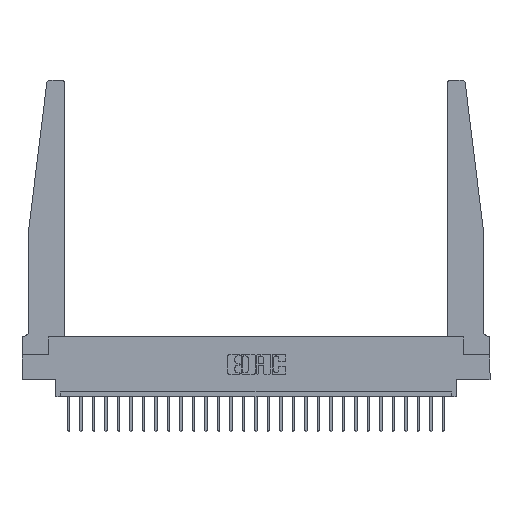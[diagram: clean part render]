
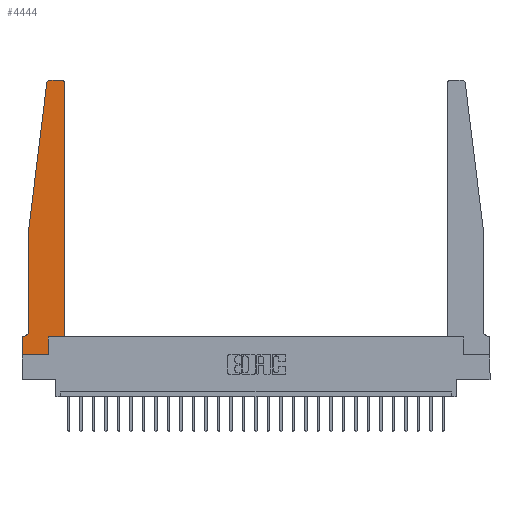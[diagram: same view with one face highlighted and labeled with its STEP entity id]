
A CAD part, top view. The second image highlights one B-rep face of the part: STEP entity #4444.
In plain terms, the highlighted planar face has unit normal (0, 0, 1).
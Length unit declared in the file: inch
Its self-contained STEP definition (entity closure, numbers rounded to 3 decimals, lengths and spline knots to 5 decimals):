
#508 = ORIENTED_EDGE ( 'NONE', *, *, #7807, .T. ) ;
#625 = EDGE_LOOP ( 'NONE', ( #10782, #24775, #23737, #12383, #6452, #21474, #19801, #24273, #508, #15521, #7440, #11717 ) ) ;
#1525 = CARTESIAN_POINT ( 'NONE',  ( 0.395, 2.72, 0.37 ) ) ;
#1667 = AXIS2_PLACEMENT_3D ( 'NONE', #6506, #8773, #2760 ) ;
#2022 = EDGE_CURVE ( 'NONE', #9186, #20017, #14570, .T. ) ;
#2147 = CARTESIAN_POINT ( 'NONE',  ( 0.27653, 2.75, 0.37 ) ) ;
#2467 = VECTOR ( 'NONE', #5396, 39.37008 ) ;
#2760 = DIRECTION ( 'NONE',  ( 1., 0., 0. ) ) ;
#2886 = AXIS2_PLACEMENT_3D ( 'NONE', #18927, #4841, #7091 ) ;
#3070 = CARTESIAN_POINT ( 'NONE',  ( 0.25, 2.75, 0.37 ) ) ;
#4006 = CARTESIAN_POINT ( 'NONE',  ( 0., 0.1875, 0.37 ) ) ;
#4007 = CARTESIAN_POINT ( 'NONE',  ( 0.015, 0.1875, 0.37 ) ) ;
#4085 = CARTESIAN_POINT ( 'NONE',  ( 0.425, 0.18, 0.37 ) ) ;
#4384 = VECTOR ( 'NONE', #7487, 39.37008 ) ;
#4444 = ADVANCED_FACE ( 'NONE', ( #12600 ), #25654, .T. ) ;
#4841 = DIRECTION ( 'NONE',  ( 0., 0., -1. ) ) ;
#5156 = EDGE_CURVE ( 'NONE', #14250, #10541, #24199, .T. ) ;
#5257 = VERTEX_POINT ( 'NONE', #4085 ) ;
#5294 = LINE ( 'NONE', #23390, #18319 ) ;
#5396 = DIRECTION ( 'NONE',  ( 0., -1., 0. ) ) ;
#5636 = EDGE_CURVE ( 'NONE', #18370, #9739, #24785, .T. ) ;
#6045 = EDGE_CURVE ( 'NONE', #23744, #9186, #22267, .T. ) ;
#6452 = ORIENTED_EDGE ( 'NONE', *, *, #2022, .T. ) ;
#6506 = CARTESIAN_POINT ( 'NONE',  ( 0.27653, 2.72, 0.37 ) ) ;
#6831 = DIRECTION ( 'NONE',  ( 0., 1., 0. ) ) ;
#7091 = DIRECTION ( 'NONE',  ( -1., 0., 0. ) ) ;
#7416 = EDGE_CURVE ( 'NONE', #20017, #22170, #16360, .T. ) ;
#7440 = ORIENTED_EDGE ( 'NONE', *, *, #16247, .T. ) ;
#7487 = DIRECTION ( 'NONE',  ( 1., 0., 0. ) ) ;
#7807 = EDGE_CURVE ( 'NONE', #10541, #13994, #12929, .T. ) ;
#7838 = DIRECTION ( 'NONE',  ( 0., 0., 1. ) ) ;
#7997 = VECTOR ( 'NONE', #18767, 39.37008 ) ;
#8141 = EDGE_CURVE ( 'NONE', #9739, #23744, #11986, .T. ) ;
#8773 = DIRECTION ( 'NONE',  ( 0., 0., 1. ) ) ;
#9186 = VERTEX_POINT ( 'NONE', #20401 ) ;
#9189 = VECTOR ( 'NONE', #20879, 39.37008 ) ;
#9529 = DIRECTION ( 'NONE',  ( 1., 0., 0. ) ) ;
#9532 = VECTOR ( 'NONE', #18486, 39.37008 ) ;
#9739 = VERTEX_POINT ( 'NONE', #24891 ) ;
#10285 = EDGE_CURVE ( 'NONE', #23157, #18370, #13423, .T. ) ;
#10321 = VECTOR ( 'NONE', #16860, 39.37008 ) ;
#10541 = VERTEX_POINT ( 'NONE', #16503 ) ;
#10782 = ORIENTED_EDGE ( 'NONE', *, *, #10285, .T. ) ;
#11386 = VERTEX_POINT ( 'NONE', #14234 ) ;
#11481 = CARTESIAN_POINT ( 'NONE',  ( 0., 0., 0.37 ) ) ;
#11717 = ORIENTED_EDGE ( 'NONE', *, *, #21036, .T. ) ;
#11986 = LINE ( 'NONE', #12971, #9189 ) ;
#12216 = CARTESIAN_POINT ( 'NONE',  ( 0., 0., 0.37 ) ) ;
#12383 = ORIENTED_EDGE ( 'NONE', *, *, #6045, .T. ) ;
#12434 = EDGE_CURVE ( 'NONE', #13994, #5257, #19121, .T. ) ;
#12557 = CARTESIAN_POINT ( 'NONE',  ( 0.2605, 0.18, 0.37 ) ) ;
#12559 = CARTESIAN_POINT ( 'NONE',  ( 0., 0.1875, 0.37 ) ) ;
#12600 = FACE_OUTER_BOUND ( 'NONE', #625, .T. ) ;
#12843 = CARTESIAN_POINT ( 'NONE',  ( 0.425, 0.18, 0.37 ) ) ;
#12929 = LINE ( 'NONE', #12557, #9532 ) ;
#12971 = CARTESIAN_POINT ( 'NONE',  ( 0.065, 1.25, 0.37 ) ) ;
#13089 = CARTESIAN_POINT ( 'NONE',  ( 0.2605, 0.18, 0.37 ) ) ;
#13346 = CARTESIAN_POINT ( 'NONE',  ( 0.065, 1.25, 0.37 ) ) ;
#13423 = LINE ( 'NONE', #3070, #10321 ) ;
#13994 = VERTEX_POINT ( 'NONE', #13089 ) ;
#14234 = CARTESIAN_POINT ( 'NONE',  ( 0.425, 2.72, 0.37 ) ) ;
#14250 = VERTEX_POINT ( 'NONE', #12216 ) ;
#14570 = CIRCLE ( 'NONE', #2886, 0.05 ) ;
#14843 = DIRECTION ( 'NONE',  ( -1., 0., 0. ) ) ;
#15164 = CARTESIAN_POINT ( 'NONE',  ( 0.395, 2.75, 0.37 ) ) ;
#15274 = CARTESIAN_POINT ( 'NONE',  ( 0.065, 1.25, 0.37 ) ) ;
#15460 = DIRECTION ( 'NONE',  ( 0., 0., 1. ) ) ;
#15521 = ORIENTED_EDGE ( 'NONE', *, *, #12434, .T. ) ;
#16247 = EDGE_CURVE ( 'NONE', #5257, #11386, #5294, .T. ) ;
#16360 = LINE ( 'NONE', #16748, #17584 ) ;
#16503 = CARTESIAN_POINT ( 'NONE',  ( 0.2605, 0., 0.37 ) ) ;
#16748 = CARTESIAN_POINT ( 'NONE',  ( 0.065, 0.1875, 0.37 ) ) ;
#16860 = DIRECTION ( 'NONE',  ( -1., 0., 0. ) ) ;
#16989 = CIRCLE ( 'NONE', #21179, 0.03 ) ;
#17584 = VECTOR ( 'NONE', #14843, 39.37008 ) ;
#18015 = AXIS2_PLACEMENT_3D ( 'NONE', #4006, #7838, #23596 ) ;
#18319 = VECTOR ( 'NONE', #6831, 39.37008 ) ;
#18370 = VERTEX_POINT ( 'NONE', #2147 ) ;
#18486 = DIRECTION ( 'NONE',  ( 0., 1., 0. ) ) ;
#18767 = DIRECTION ( 'NONE',  ( 1., 0., 0. ) ) ;
#18927 = CARTESIAN_POINT ( 'NONE',  ( 0.015, 0.2375, 0.37 ) ) ;
#19121 = LINE ( 'NONE', #12843, #7997 ) ;
#19801 = ORIENTED_EDGE ( 'NONE', *, *, #23864, .T. ) ;
#20017 = VERTEX_POINT ( 'NONE', #4007 ) ;
#20234 = VECTOR ( 'NONE', #23869, 39.37008 ) ;
#20401 = CARTESIAN_POINT ( 'NONE',  ( 0.065, 0.2375, 0.37 ) ) ;
#20556 = LINE ( 'NONE', #23787, #20234 ) ;
#20879 = DIRECTION ( 'NONE',  ( -0.122, -0.992, 0. ) ) ;
#21036 = EDGE_CURVE ( 'NONE', #11386, #23157, #16989, .T. ) ;
#21179 = AXIS2_PLACEMENT_3D ( 'NONE', #1525, #15460, #9529 ) ;
#21474 = ORIENTED_EDGE ( 'NONE', *, *, #7416, .T. ) ;
#22170 = VERTEX_POINT ( 'NONE', #12559 ) ;
#22267 = LINE ( 'NONE', #15274, #2467 ) ;
#23157 = VERTEX_POINT ( 'NONE', #15164 ) ;
#23390 = CARTESIAN_POINT ( 'NONE',  ( 0.425, 0.18, 0.37 ) ) ;
#23596 = DIRECTION ( 'NONE',  ( 1., 0., 0. ) ) ;
#23737 = ORIENTED_EDGE ( 'NONE', *, *, #8141, .T. ) ;
#23744 = VERTEX_POINT ( 'NONE', #13346 ) ;
#23787 = CARTESIAN_POINT ( 'NONE',  ( 0., 0., 0.37 ) ) ;
#23864 = EDGE_CURVE ( 'NONE', #22170, #14250, #20556, .T. ) ;
#23869 = DIRECTION ( 'NONE',  ( 0., -1., 0. ) ) ;
#24199 = LINE ( 'NONE', #11481, #4384 ) ;
#24273 = ORIENTED_EDGE ( 'NONE', *, *, #5156, .T. ) ;
#24775 = ORIENTED_EDGE ( 'NONE', *, *, #5636, .T. ) ;
#24785 = CIRCLE ( 'NONE', #1667, 0.03 ) ;
#24891 = CARTESIAN_POINT ( 'NONE',  ( 0.24675, 2.72367, 0.37 ) ) ;
#25654 = PLANE ( 'NONE',  #18015 ) ;
